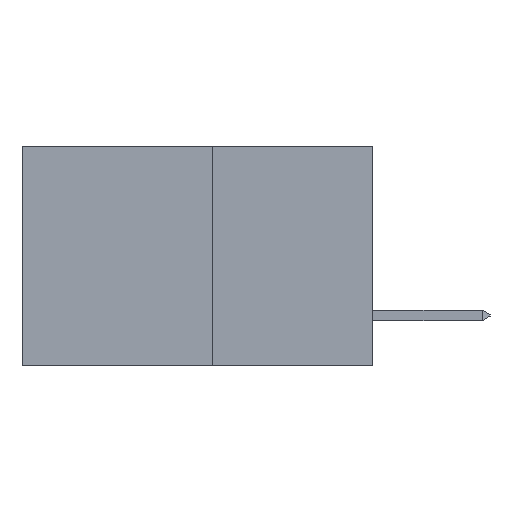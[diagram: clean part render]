
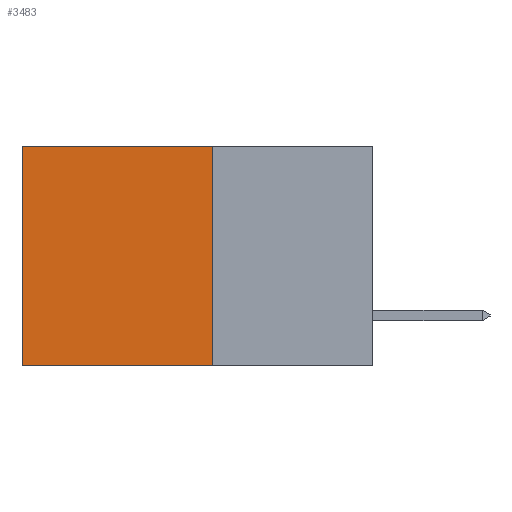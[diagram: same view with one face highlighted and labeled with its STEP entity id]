
A CAD part, left-side view. The second image highlights one B-rep face of the part: STEP entity #3483.
In plain terms, the highlighted planar face has unit normal (-1, 0, 0).
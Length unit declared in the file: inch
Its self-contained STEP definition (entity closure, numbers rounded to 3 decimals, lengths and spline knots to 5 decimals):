
#4 = CARTESIAN_POINT ( 'NONE',  ( 0.277, 0.59, -0.37 ) ) ;
#2020 = FACE_OUTER_BOUND ( 'NONE', #7734, .T. ) ;
#2185 = LINE ( 'NONE', #5786, #19740 ) ;
#3483 = ADVANCED_FACE ( 'NONE', ( #2020 ), #7392, .F. ) ;
#3992 = VERTEX_POINT ( 'NONE', #6915 ) ;
#4190 = CARTESIAN_POINT ( 'NONE',  ( 0.277, 0.59, -0.37 ) ) ;
#4205 = DIRECTION ( 'NONE',  ( 1., 0., 0. ) ) ;
#4229 = DIRECTION ( 'NONE',  ( 0., 0., -1. ) ) ;
#4251 = LINE ( 'NONE', #19900, #27729 ) ;
#4325 = LINE ( 'NONE', #4, #27796 ) ;
#4707 = CARTESIAN_POINT ( 'NONE',  ( 0.277, 0.27, -0.37 ) ) ;
#5786 = CARTESIAN_POINT ( 'NONE',  ( 0.277, 0.27, -0.37 ) ) ;
#6776 = CARTESIAN_POINT ( 'NONE',  ( 0.277, 0.27, -0.37 ) ) ;
#6915 = CARTESIAN_POINT ( 'NONE',  ( 0.277, 0.59, 0. ) ) ;
#7392 = PLANE ( 'NONE',  #14122 ) ;
#7734 = EDGE_LOOP ( 'NONE', ( #17146, #20019, #27423, #9999 ) ) ;
#8859 = EDGE_CURVE ( 'NONE', #25366, #17524, #4251, .T. ) ;
#9999 = ORIENTED_EDGE ( 'NONE', *, *, #16058, .T. ) ;
#11597 = DIRECTION ( 'NONE',  ( 0., 0., -1. ) ) ;
#12434 = EDGE_CURVE ( 'NONE', #17524, #24419, #2185, .T. ) ;
#12759 = EDGE_CURVE ( 'NONE', #3992, #24419, #4325, .T. ) ;
#14122 = AXIS2_PLACEMENT_3D ( 'NONE', #4707, #4205, #4229 ) ;
#15038 = DIRECTION ( 'NONE',  ( 0., 1., 0. ) ) ;
#16058 = EDGE_CURVE ( 'NONE', #25366, #3992, #20270, .T. ) ;
#17146 = ORIENTED_EDGE ( 'NONE', *, *, #12759, .T. ) ;
#17524 = VERTEX_POINT ( 'NONE', #6776 ) ;
#17762 = CARTESIAN_POINT ( 'NONE',  ( 0.277, 0.27, 0. ) ) ;
#19552 = VECTOR ( 'NONE', #20069, 39.37008 ) ;
#19740 = VECTOR ( 'NONE', #15038, 39.37008 ) ;
#19900 = CARTESIAN_POINT ( 'NONE',  ( 0.277, 0.27, -0.37 ) ) ;
#20019 = ORIENTED_EDGE ( 'NONE', *, *, #12434, .F. ) ;
#20069 = DIRECTION ( 'NONE',  ( 0., 1., 0. ) ) ;
#20270 = LINE ( 'NONE', #17762, #19552 ) ;
#22173 = DIRECTION ( 'NONE',  ( 0., 0., -1. ) ) ;
#23724 = CARTESIAN_POINT ( 'NONE',  ( 0.277, 0.27, 0. ) ) ;
#24419 = VERTEX_POINT ( 'NONE', #4190 ) ;
#25366 = VERTEX_POINT ( 'NONE', #23724 ) ;
#27423 = ORIENTED_EDGE ( 'NONE', *, *, #8859, .F. ) ;
#27729 = VECTOR ( 'NONE', #22173, 39.37008 ) ;
#27796 = VECTOR ( 'NONE', #11597, 39.37008 ) ;
